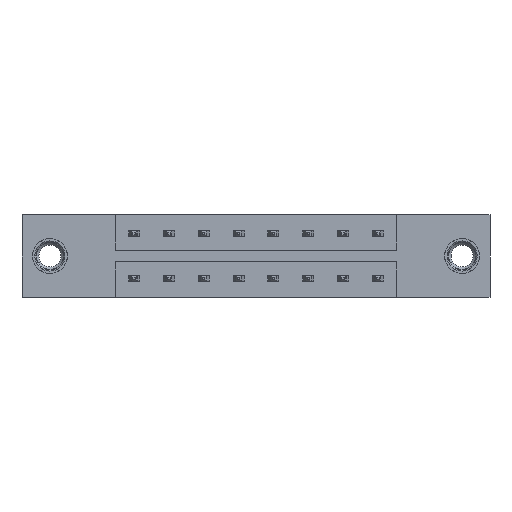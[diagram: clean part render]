
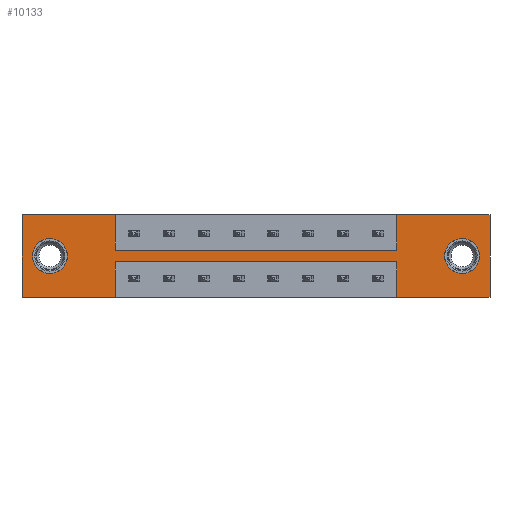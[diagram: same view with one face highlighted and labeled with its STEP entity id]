
A CAD part, front view. The second image highlights one B-rep face of the part: STEP entity #10133.
In plain terms, the highlighted planar face has unit normal (0, -1, 0).
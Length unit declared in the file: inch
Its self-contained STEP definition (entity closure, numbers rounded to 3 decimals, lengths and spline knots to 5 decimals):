
#123 = CIRCLE ( 'NONE', #3112, 0.078 ) ;
#196 = CARTESIAN_POINT ( 'NONE',  ( 0.4175, 0., -0.2115 ) ) ;
#214 = CARTESIAN_POINT ( 'NONE',  ( 0.125, 0., -0.263 ) ) ;
#463 = VECTOR ( 'NONE', #7841, 39.37008 ) ;
#558 = CARTESIAN_POINT ( 'NONE',  ( 1.6785, 0., -0.37 ) ) ;
#631 = DIRECTION ( 'NONE',  ( 1., 0., 0. ) ) ;
#655 = CARTESIAN_POINT ( 'NONE',  ( 0.4175, 0., -0.37 ) ) ;
#725 = EDGE_CURVE ( 'NONE', #5999, #5480, #6002, .T. ) ;
#750 = EDGE_CURVE ( 'NONE', #6476, #5999, #4209, .T. ) ;
#818 = DIRECTION ( 'NONE',  ( 0., 0., -1. ) ) ;
#937 = CIRCLE ( 'NONE', #3034, 0.078 ) ;
#986 = CARTESIAN_POINT ( 'NONE',  ( 0.125, 0., -0.185 ) ) ;
#994 = CARTESIAN_POINT ( 'NONE',  ( 2.096, 0., -0.37 ) ) ;
#1084 = VECTOR ( 'NONE', #9294, 39.37008 ) ;
#1308 = AXIS2_PLACEMENT_3D ( 'NONE', #1408, #2183, #7936 ) ;
#1408 = CARTESIAN_POINT ( 'NONE',  ( 0., 0., -0.37 ) ) ;
#1448 = EDGE_LOOP ( 'NONE', ( #5880, #5031, #4028, #2475, #5801, #9795, #9801, #9330, #9711, #5341, #1799, #3844 ) ) ;
#1574 = EDGE_CURVE ( 'NONE', #9982, #5841, #937, .T. ) ;
#1619 = LINE ( 'NONE', #4970, #10614 ) ;
#1792 = VECTOR ( 'NONE', #8456, 39.37008 ) ;
#1799 = ORIENTED_EDGE ( 'NONE', *, *, #750, .F. ) ;
#1867 = EDGE_LOOP ( 'NONE', ( #3218, #9874 ) ) ;
#2020 = CARTESIAN_POINT ( 'NONE',  ( 0., 0., -0.37 ) ) ;
#2079 = PLANE ( 'NONE',  #1308 ) ;
#2155 = VECTOR ( 'NONE', #6903, 39.37008 ) ;
#2183 = DIRECTION ( 'NONE',  ( 0., -1., 0. ) ) ;
#2375 = LINE ( 'NONE', #4848, #8066 ) ;
#2389 = LINE ( 'NONE', #5727, #463 ) ;
#2475 = ORIENTED_EDGE ( 'NONE', *, *, #4067, .F. ) ;
#2558 = CARTESIAN_POINT ( 'NONE',  ( 0., 0., 0. ) ) ;
#2569 = VERTEX_POINT ( 'NONE', #2558 ) ;
#2691 = DIRECTION ( 'NONE',  ( 0., 0., 1. ) ) ;
#2788 = VERTEX_POINT ( 'NONE', #3803 ) ;
#2894 = EDGE_CURVE ( 'NONE', #4192, #7365, #2375, .T. ) ;
#2988 = CARTESIAN_POINT ( 'NONE',  ( 0.125, 0., -0.185 ) ) ;
#3003 = LINE ( 'NONE', #10334, #7028 ) ;
#3034 = AXIS2_PLACEMENT_3D ( 'NONE', #2988, #6289, #4791 ) ;
#3112 = AXIS2_PLACEMENT_3D ( 'NONE', #4413, #7741, #10315 ) ;
#3218 = ORIENTED_EDGE ( 'NONE', *, *, #9585, .T. ) ;
#3295 = CARTESIAN_POINT ( 'NONE',  ( 1.971, 0., -0.185 ) ) ;
#3489 = CARTESIAN_POINT ( 'NONE',  ( 1.6785, 0., 0. ) ) ;
#3712 = DIRECTION ( 'NONE',  ( 0., 0., -1. ) ) ;
#3726 = VECTOR ( 'NONE', #9474, 39.37008 ) ;
#3803 = CARTESIAN_POINT ( 'NONE',  ( 1.971, 0., -0.107 ) ) ;
#3806 = LINE ( 'NONE', #7314, #10205 ) ;
#3835 = FACE_BOUND ( 'NONE', #1867, .T. ) ;
#3844 = ORIENTED_EDGE ( 'NONE', *, *, #3991, .F. ) ;
#3870 = EDGE_CURVE ( 'NONE', #6854, #2788, #5657, .T. ) ;
#3991 = EDGE_CURVE ( 'NONE', #4113, #6476, #4381, .T. ) ;
#4028 = ORIENTED_EDGE ( 'NONE', *, *, #4114, .F. ) ;
#4067 = EDGE_CURVE ( 'NONE', #7365, #4604, #6415, .T. ) ;
#4083 = EDGE_LOOP ( 'NONE', ( #9819, #4784 ) ) ;
#4112 = EDGE_CURVE ( 'NONE', #10394, #9965, #10441, .T. ) ;
#4113 = VERTEX_POINT ( 'NONE', #9519 ) ;
#4114 = EDGE_CURVE ( 'NONE', #4604, #5740, #3003, .T. ) ;
#4154 = DIRECTION ( 'NONE',  ( 0., 0., 1. ) ) ;
#4192 = VERTEX_POINT ( 'NONE', #4806 ) ;
#4209 = LINE ( 'NONE', #10073, #1084 ) ;
#4323 = DIRECTION ( 'NONE',  ( 1., 0., 0. ) ) ;
#4381 = LINE ( 'NONE', #196, #2155 ) ;
#4413 = CARTESIAN_POINT ( 'NONE',  ( 1.971, 0., -0.185 ) ) ;
#4477 = CARTESIAN_POINT ( 'NONE',  ( 1.971, 0., -0.263 ) ) ;
#4487 = VERTEX_POINT ( 'NONE', #558 ) ;
#4517 = LINE ( 'NONE', #5125, #9508 ) ;
#4604 = VERTEX_POINT ( 'NONE', #8212 ) ;
#4608 = FACE_OUTER_BOUND ( 'NONE', #1448, .T. ) ;
#4752 = DIRECTION ( 'NONE',  ( 1., 0., 0. ) ) ;
#4784 = ORIENTED_EDGE ( 'NONE', *, *, #10466, .T. ) ;
#4791 = DIRECTION ( 'NONE',  ( 0., 0., 1. ) ) ;
#4806 = CARTESIAN_POINT ( 'NONE',  ( 1.6785, 0., -0.1585 ) ) ;
#4848 = CARTESIAN_POINT ( 'NONE',  ( 1.6785, 0., -0.1585 ) ) ;
#4970 = CARTESIAN_POINT ( 'NONE',  ( 1.6785, 0., -0.2115 ) ) ;
#4974 = DIRECTION ( 'NONE',  ( 0., 1., 0. ) ) ;
#5031 = ORIENTED_EDGE ( 'NONE', *, *, #10573, .F. ) ;
#5125 = CARTESIAN_POINT ( 'NONE',  ( 0.4175, 0., -0.1585 ) ) ;
#5183 = CARTESIAN_POINT ( 'NONE',  ( 0., 0., -0.37 ) ) ;
#5250 = CARTESIAN_POINT ( 'NONE',  ( 0.4175, 0., 0. ) ) ;
#5261 = CARTESIAN_POINT ( 'NONE',  ( 0.4175, 0., -0.1585 ) ) ;
#5341 = ORIENTED_EDGE ( 'NONE', *, *, #725, .F. ) ;
#5371 = CARTESIAN_POINT ( 'NONE',  ( 0.125, 0., -0.107 ) ) ;
#5423 = EDGE_CURVE ( 'NONE', #5480, #2569, #2389, .T. ) ;
#5452 = CARTESIAN_POINT ( 'NONE',  ( 0.4175, 0., -0.1585 ) ) ;
#5480 = VERTEX_POINT ( 'NONE', #8765 ) ;
#5563 = EDGE_CURVE ( 'NONE', #9965, #4192, #4517, .T. ) ;
#5657 = CIRCLE ( 'NONE', #9822, 0.078 ) ;
#5662 = VECTOR ( 'NONE', #3712, 39.37008 ) ;
#5710 = DIRECTION ( 'NONE',  ( 0., 0., 1. ) ) ;
#5727 = CARTESIAN_POINT ( 'NONE',  ( 0., 0., 0. ) ) ;
#5740 = VERTEX_POINT ( 'NONE', #994 ) ;
#5801 = ORIENTED_EDGE ( 'NONE', *, *, #2894, .F. ) ;
#5841 = VERTEX_POINT ( 'NONE', #214 ) ;
#5880 = ORIENTED_EDGE ( 'NONE', *, *, #8197, .F. ) ;
#5999 = VERTEX_POINT ( 'NONE', #655 ) ;
#6002 = LINE ( 'NONE', #5183, #1792 ) ;
#6289 = DIRECTION ( 'NONE',  ( 0., 1., 0. ) ) ;
#6415 = LINE ( 'NONE', #9684, #9467 ) ;
#6476 = VERTEX_POINT ( 'NONE', #8734 ) ;
#6854 = VERTEX_POINT ( 'NONE', #4477 ) ;
#6903 = DIRECTION ( 'NONE',  ( -1., 0., 0. ) ) ;
#7028 = VECTOR ( 'NONE', #8727, 39.37008 ) ;
#7314 = CARTESIAN_POINT ( 'NONE',  ( 0., 0., 0. ) ) ;
#7365 = VERTEX_POINT ( 'NONE', #3489 ) ;
#7741 = DIRECTION ( 'NONE',  ( 0., 1., 0. ) ) ;
#7841 = DIRECTION ( 'NONE',  ( 0., 0., 1. ) ) ;
#7936 = DIRECTION ( 'NONE',  ( 0., 0., -1. ) ) ;
#8066 = VECTOR ( 'NONE', #5710, 39.37008 ) ;
#8197 = EDGE_CURVE ( 'NONE', #4487, #4113, #1619, .T. ) ;
#8212 = CARTESIAN_POINT ( 'NONE',  ( 2.096, 0., 0. ) ) ;
#8456 = DIRECTION ( 'NONE',  ( -1., 0., 0. ) ) ;
#8727 = DIRECTION ( 'NONE',  ( 0., 0., -1. ) ) ;
#8734 = CARTESIAN_POINT ( 'NONE',  ( 0.4175, 0., -0.2115 ) ) ;
#8765 = CARTESIAN_POINT ( 'NONE',  ( 0., 0., -0.37 ) ) ;
#8852 = FACE_BOUND ( 'NONE', #4083, .T. ) ;
#9284 = AXIS2_PLACEMENT_3D ( 'NONE', #986, #9310, #2691 ) ;
#9294 = DIRECTION ( 'NONE',  ( 0., 0., -1. ) ) ;
#9310 = DIRECTION ( 'NONE',  ( 0., 1., 0. ) ) ;
#9320 = EDGE_CURVE ( 'NONE', #2569, #10394, #3806, .T. ) ;
#9330 = ORIENTED_EDGE ( 'NONE', *, *, #9320, .F. ) ;
#9454 = CIRCLE ( 'NONE', #9284, 0.078 ) ;
#9467 = VECTOR ( 'NONE', #4752, 39.37008 ) ;
#9474 = DIRECTION ( 'NONE',  ( -1., 0., 0. ) ) ;
#9508 = VECTOR ( 'NONE', #4323, 39.37008 ) ;
#9519 = CARTESIAN_POINT ( 'NONE',  ( 1.6785, 0., -0.2115 ) ) ;
#9528 = LINE ( 'NONE', #2020, #3726 ) ;
#9585 = EDGE_CURVE ( 'NONE', #2788, #6854, #123, .T. ) ;
#9684 = CARTESIAN_POINT ( 'NONE',  ( 0., 0., 0. ) ) ;
#9711 = ORIENTED_EDGE ( 'NONE', *, *, #5423, .F. ) ;
#9795 = ORIENTED_EDGE ( 'NONE', *, *, #5563, .F. ) ;
#9801 = ORIENTED_EDGE ( 'NONE', *, *, #4112, .F. ) ;
#9819 = ORIENTED_EDGE ( 'NONE', *, *, #1574, .T. ) ;
#9822 = AXIS2_PLACEMENT_3D ( 'NONE', #3295, #4974, #818 ) ;
#9874 = ORIENTED_EDGE ( 'NONE', *, *, #3870, .T. ) ;
#9965 = VERTEX_POINT ( 'NONE', #5261 ) ;
#9982 = VERTEX_POINT ( 'NONE', #5371 ) ;
#10073 = CARTESIAN_POINT ( 'NONE',  ( 0.4175, 0., -0.2115 ) ) ;
#10133 = ADVANCED_FACE ( 'NONE', ( #3835, #8852, #4608 ), #2079, .T. ) ;
#10205 = VECTOR ( 'NONE', #631, 39.37008 ) ;
#10315 = DIRECTION ( 'NONE',  ( 0., 0., -1. ) ) ;
#10334 = CARTESIAN_POINT ( 'NONE',  ( 2.096, 0., 0. ) ) ;
#10394 = VERTEX_POINT ( 'NONE', #5250 ) ;
#10441 = LINE ( 'NONE', #5452, #5662 ) ;
#10466 = EDGE_CURVE ( 'NONE', #5841, #9982, #9454, .T. ) ;
#10573 = EDGE_CURVE ( 'NONE', #5740, #4487, #9528, .T. ) ;
#10614 = VECTOR ( 'NONE', #4154, 39.37008 ) ;
